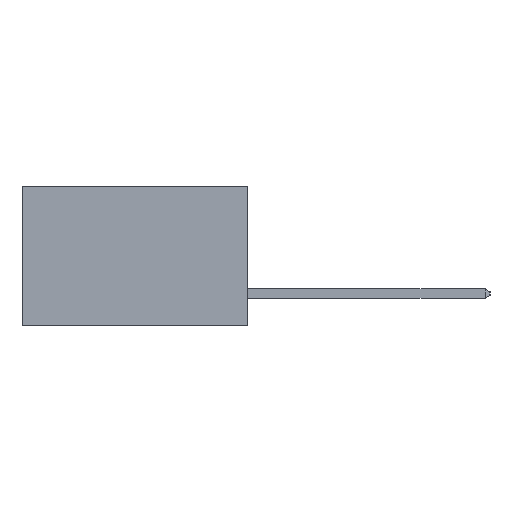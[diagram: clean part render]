
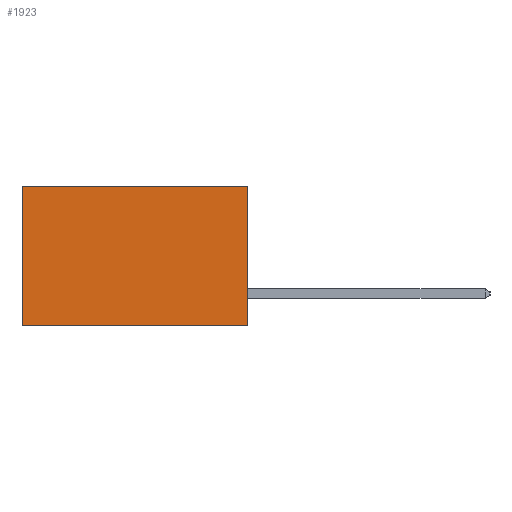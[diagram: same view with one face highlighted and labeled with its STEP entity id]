
A CAD part, left-side view. The second image highlights one B-rep face of the part: STEP entity #1923.
In plain terms, the highlighted planar face has unit normal (-1, 0, 0).
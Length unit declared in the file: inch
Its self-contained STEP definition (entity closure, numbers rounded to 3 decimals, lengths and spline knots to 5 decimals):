
#439 = EDGE_CURVE ( 'NONE', #2595, #13163, #2018, .T. ) ;
#1010 = ORIENTED_EDGE ( 'NONE', *, *, #2603, .F. ) ;
#1243 = VERTEX_POINT ( 'NONE', #9065 ) ;
#1324 = FACE_OUTER_BOUND ( 'NONE', #12970, .T. ) ;
#1809 = DIRECTION ( 'NONE',  ( 0., 0., -1. ) ) ;
#1923 = ADVANCED_FACE ( 'NONE', ( #1324 ), #11021, .F. ) ;
#2018 = LINE ( 'NONE', #8422, #2719 ) ;
#2019 = VERTEX_POINT ( 'NONE', #9996 ) ;
#2595 = VERTEX_POINT ( 'NONE', #11221 ) ;
#2603 = EDGE_CURVE ( 'NONE', #2019, #2595, #12529, .T. ) ;
#2719 = VECTOR ( 'NONE', #13823, 39.37008 ) ;
#2885 = AXIS2_PLACEMENT_3D ( 'NONE', #9813, #10966, #5554 ) ;
#3035 = CARTESIAN_POINT ( 'NONE',  ( 0.2615, 0.6, -0.37 ) ) ;
#4421 = LINE ( 'NONE', #3035, #9807 ) ;
#5055 = ORIENTED_EDGE ( 'NONE', *, *, #439, .F. ) ;
#5554 = DIRECTION ( 'NONE',  ( 0., 0., -1. ) ) ;
#6143 = VECTOR ( 'NONE', #11124, 39.37008 ) ;
#6583 = EDGE_CURVE ( 'NONE', #1243, #13163, #4421, .T. ) ;
#8422 = CARTESIAN_POINT ( 'NONE',  ( 0.2615, 0., -0.37 ) ) ;
#9065 = CARTESIAN_POINT ( 'NONE',  ( 0.2615, 0.6, 0. ) ) ;
#9217 = DIRECTION ( 'NONE',  ( 0., 1., 0. ) ) ;
#9261 = CARTESIAN_POINT ( 'NONE',  ( 0.2615, 0., 0. ) ) ;
#9807 = VECTOR ( 'NONE', #1809, 39.37008 ) ;
#9813 = CARTESIAN_POINT ( 'NONE',  ( 0.2615, 0., -0.37 ) ) ;
#9887 = EDGE_CURVE ( 'NONE', #2019, #1243, #13694, .T. ) ;
#9996 = CARTESIAN_POINT ( 'NONE',  ( 0.2615, 0., 0. ) ) ;
#10168 = CARTESIAN_POINT ( 'NONE',  ( 0.2615, 0.6, -0.37 ) ) ;
#10966 = DIRECTION ( 'NONE',  ( 1., 0., 0. ) ) ;
#11021 = PLANE ( 'NONE',  #2885 ) ;
#11057 = ORIENTED_EDGE ( 'NONE', *, *, #6583, .T. ) ;
#11124 = DIRECTION ( 'NONE',  ( 0., 0., -1. ) ) ;
#11174 = CARTESIAN_POINT ( 'NONE',  ( 0.2615, 0., -0.37 ) ) ;
#11221 = CARTESIAN_POINT ( 'NONE',  ( 0.2615, 0., -0.37 ) ) ;
#12529 = LINE ( 'NONE', #11174, #6143 ) ;
#12970 = EDGE_LOOP ( 'NONE', ( #11057, #5055, #1010, #13199 ) ) ;
#13031 = VECTOR ( 'NONE', #9217, 39.37008 ) ;
#13163 = VERTEX_POINT ( 'NONE', #10168 ) ;
#13199 = ORIENTED_EDGE ( 'NONE', *, *, #9887, .T. ) ;
#13694 = LINE ( 'NONE', #9261, #13031 ) ;
#13823 = DIRECTION ( 'NONE',  ( 0., 1., 0. ) ) ;
